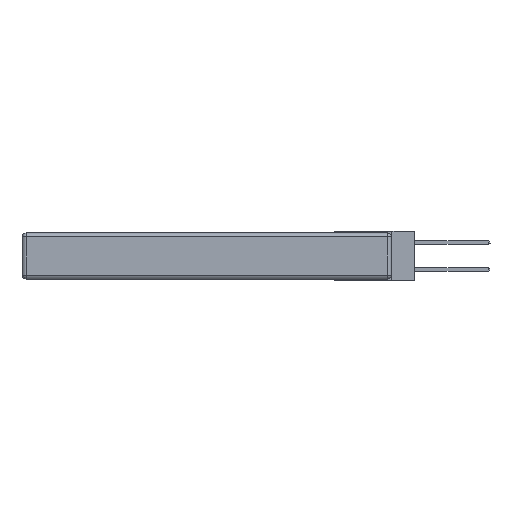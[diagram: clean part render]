
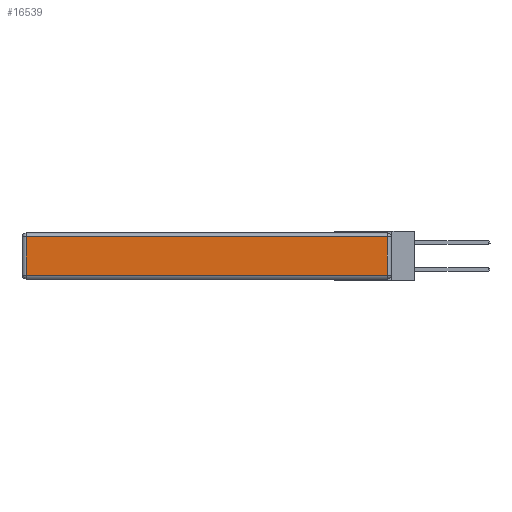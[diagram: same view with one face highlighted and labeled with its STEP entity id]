
A CAD part, left-side view. The second image highlights one B-rep face of the part: STEP entity #16539.
In plain terms, the highlighted planar face has unit normal (-1, 0, 0).
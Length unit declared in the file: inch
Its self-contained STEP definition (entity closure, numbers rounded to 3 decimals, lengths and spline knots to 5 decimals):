
#636 = DIRECTION ( 'NONE',  ( 0., 0., 1. ) ) ;
#1148 = ORIENTED_EDGE ( 'NONE', *, *, #10090, .T. ) ;
#1648 = CARTESIAN_POINT ( 'NONE',  ( 0., 2.72, -0.313 ) ) ;
#2670 = CARTESIAN_POINT ( 'NONE',  ( 0., 0.03, -0.03 ) ) ;
#2799 = VECTOR ( 'NONE', #7783, 39.37008 ) ;
#2907 = CARTESIAN_POINT ( 'NONE',  ( 0., 0., -0.313 ) ) ;
#4110 = DIRECTION ( 'NONE',  ( 0., -1., 0. ) ) ;
#4895 = ORIENTED_EDGE ( 'NONE', *, *, #5701, .T. ) ;
#5701 = EDGE_CURVE ( 'NONE', #16050, #11488, #11635, .T. ) ;
#5705 = VERTEX_POINT ( 'NONE', #6397 ) ;
#5857 = CARTESIAN_POINT ( 'NONE',  ( 0., 2.72, -0.03 ) ) ;
#6339 = LINE ( 'NONE', #12010, #2799 ) ;
#6397 = CARTESIAN_POINT ( 'NONE',  ( 0., 0.03, -0.313 ) ) ;
#7320 = VERTEX_POINT ( 'NONE', #1648 ) ;
#7353 = PLANE ( 'NONE',  #8450 ) ;
#7411 = DIRECTION ( 'NONE',  ( -1., 0., 0. ) ) ;
#7783 = DIRECTION ( 'NONE',  ( 0., 0., -1. ) ) ;
#8450 = AXIS2_PLACEMENT_3D ( 'NONE', #11353, #7411, #636 ) ;
#8851 = LINE ( 'NONE', #9348, #15206 ) ;
#9348 = CARTESIAN_POINT ( 'NONE',  ( 0., 0.03, -0.343 ) ) ;
#9501 = VECTOR ( 'NONE', #16013, 39.37008 ) ;
#10090 = EDGE_CURVE ( 'NONE', #7320, #5705, #11485, .T. ) ;
#10632 = VECTOR ( 'NONE', #4110, 39.37008 ) ;
#10681 = EDGE_LOOP ( 'NONE', ( #1148, #11114, #4895, #14355 ) ) ;
#11114 = ORIENTED_EDGE ( 'NONE', *, *, #11975, .T. ) ;
#11353 = CARTESIAN_POINT ( 'NONE',  ( 0., 0., -0.343 ) ) ;
#11485 = LINE ( 'NONE', #2907, #10632 ) ;
#11488 = VERTEX_POINT ( 'NONE', #5857 ) ;
#11635 = LINE ( 'NONE', #14470, #9501 ) ;
#11975 = EDGE_CURVE ( 'NONE', #5705, #16050, #8851, .T. ) ;
#12010 = CARTESIAN_POINT ( 'NONE',  ( 0., 2.72, -0.343 ) ) ;
#12189 = FACE_OUTER_BOUND ( 'NONE', #10681, .T. ) ;
#14355 = ORIENTED_EDGE ( 'NONE', *, *, #15889, .T. ) ;
#14470 = CARTESIAN_POINT ( 'NONE',  ( 0., 2.75, -0.03 ) ) ;
#14735 = DIRECTION ( 'NONE',  ( 0., 0., 1. ) ) ;
#15206 = VECTOR ( 'NONE', #14735, 39.37008 ) ;
#15889 = EDGE_CURVE ( 'NONE', #11488, #7320, #6339, .T. ) ;
#16013 = DIRECTION ( 'NONE',  ( 0., 1., 0. ) ) ;
#16050 = VERTEX_POINT ( 'NONE', #2670 ) ;
#16539 = ADVANCED_FACE ( 'NONE', ( #12189 ), #7353, .T. ) ;
